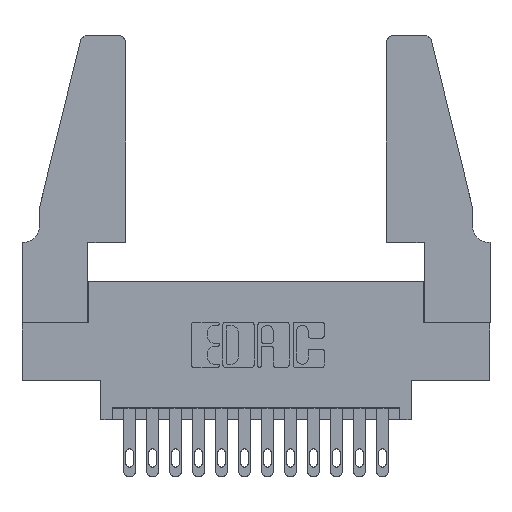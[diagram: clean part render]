
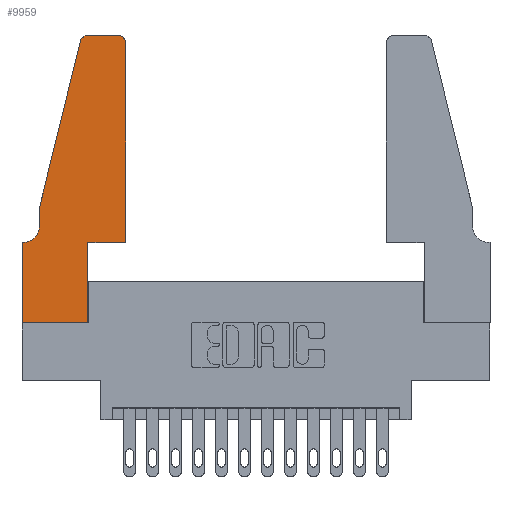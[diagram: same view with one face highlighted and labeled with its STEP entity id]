
A CAD part, top view. The second image highlights one B-rep face of the part: STEP entity #9959.
In plain terms, the highlighted planar face has unit normal (0, 0, 1).
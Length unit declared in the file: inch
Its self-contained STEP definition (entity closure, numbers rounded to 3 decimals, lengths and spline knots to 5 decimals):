
#81 = EDGE_CURVE ( 'NONE', #7477, #2497, #8953, .T. ) ;
#582 = ORIENTED_EDGE ( 'NONE', *, *, #3289, .T. ) ;
#602 = ORIENTED_EDGE ( 'NONE', *, *, #713, .T. ) ;
#713 = EDGE_CURVE ( 'NONE', #14682, #7477, #11780, .T. ) ;
#714 = PLANE ( 'NONE',  #820 ) ;
#746 = LINE ( 'NONE', #6667, #15340 ) ;
#820 = AXIS2_PLACEMENT_3D ( 'NONE', #15284, #14021, #11744 ) ;
#969 = DIRECTION ( 'NONE',  ( 1., 0., 0. ) ) ;
#1720 = CARTESIAN_POINT ( 'NONE',  ( 0.0055, 0.42, 0.37 ) ) ;
#1726 = CARTESIAN_POINT ( 'NONE',  ( 0.2865, 0.35, 0.37 ) ) ;
#1733 = EDGE_CURVE ( 'NONE', #10655, #14813, #12860, .T. ) ;
#1747 = ORIENTED_EDGE ( 'NONE', *, *, #14807, .T. ) ;
#1910 = CIRCLE ( 'NONE', #2543, 0.03 ) ;
#1950 = FACE_OUTER_BOUND ( 'NONE', #2334, .T. ) ;
#2334 = EDGE_LOOP ( 'NONE', ( #6876, #14198, #11317, #602, #5118, #5185, #582, #6405, #6562, #12380, #1747, #8671 ) ) ;
#2339 = VERTEX_POINT ( 'NONE', #14355 ) ;
#2362 = DIRECTION ( 'NONE',  ( 1., 0., 0. ) ) ;
#2379 = EDGE_CURVE ( 'NONE', #2339, #4622, #3579, .T. ) ;
#2497 = VERTEX_POINT ( 'NONE', #14504 ) ;
#2543 = AXIS2_PLACEMENT_3D ( 'NONE', #4856, #8534, #2362 ) ;
#2644 = VECTOR ( 'NONE', #969, 39.37008 ) ;
#3289 = EDGE_CURVE ( 'NONE', #13459, #10655, #746, .T. ) ;
#3384 = LINE ( 'NONE', #5779, #15113 ) ;
#3412 = DIRECTION ( 'NONE',  ( -1., 0., 0. ) ) ;
#3437 = VECTOR ( 'NONE', #10506, 39.37008 ) ;
#3526 = EDGE_CURVE ( 'NONE', #9726, #8378, #5277, .T. ) ;
#3579 = CIRCLE ( 'NONE', #4833, 0.03 ) ;
#3986 = CARTESIAN_POINT ( 'NONE',  ( 0.0755, 0.42, 0.37 ) ) ;
#4255 = LINE ( 'NONE', #6938, #6357 ) ;
#4392 = DIRECTION ( 'NONE',  ( 1., 0., 0. ) ) ;
#4622 = VERTEX_POINT ( 'NONE', #6250 ) ;
#4772 = CARTESIAN_POINT ( 'NONE',  ( 0.4505, 0.35, 0.37 ) ) ;
#4833 = AXIS2_PLACEMENT_3D ( 'NONE', #8359, #11648, #4392 ) ;
#4856 = CARTESIAN_POINT ( 'NONE',  ( 0.284, 1.22, 0.37 ) ) ;
#5118 = ORIENTED_EDGE ( 'NONE', *, *, #81, .T. ) ;
#5185 = ORIENTED_EDGE ( 'NONE', *, *, #6138, .T. ) ;
#5277 = LINE ( 'NONE', #6906, #11356 ) ;
#5686 = DIRECTION ( 'NONE',  ( 0., -1., 0. ) ) ;
#5779 = CARTESIAN_POINT ( 'NONE',  ( 0.2605, 1.25, 0.37 ) ) ;
#5795 = CARTESIAN_POINT ( 'NONE',  ( 0., 0., 0.37 ) ) ;
#5991 = LINE ( 'NONE', #15355, #14851 ) ;
#5999 = DIRECTION ( 'NONE',  ( 0., 1., 0. ) ) ;
#6138 = EDGE_CURVE ( 'NONE', #2497, #13459, #5991, .T. ) ;
#6250 = CARTESIAN_POINT ( 'NONE',  ( 0.4205, 1.25, 0.37 ) ) ;
#6342 = EDGE_CURVE ( 'NONE', #13863, #14682, #4255, .T. ) ;
#6357 = VECTOR ( 'NONE', #10728, 39.37008 ) ;
#6405 = ORIENTED_EDGE ( 'NONE', *, *, #1733, .T. ) ;
#6513 = DIRECTION ( 'NONE',  ( 0., 1., 0. ) ) ;
#6562 = ORIENTED_EDGE ( 'NONE', *, *, #8147, .T. ) ;
#6667 = CARTESIAN_POINT ( 'NONE',  ( 0., 0., 0.37 ) ) ;
#6869 = CARTESIAN_POINT ( 'NONE',  ( 0.2865, 0., 0.37 ) ) ;
#6876 = ORIENTED_EDGE ( 'NONE', *, *, #13393, .T. ) ;
#6906 = CARTESIAN_POINT ( 'NONE',  ( 0.4505, 0.35, 0.37 ) ) ;
#6938 = CARTESIAN_POINT ( 'NONE',  ( 0.0755, 0.5, 0.37 ) ) ;
#6979 = CARTESIAN_POINT ( 'NONE',  ( 0.2865, 0.35, 0.37 ) ) ;
#7275 = AXIS2_PLACEMENT_3D ( 'NONE', #1720, #10667, #3412 ) ;
#7477 = VERTEX_POINT ( 'NONE', #3986 ) ;
#7820 = LINE ( 'NONE', #1726, #13453 ) ;
#8109 = VERTEX_POINT ( 'NONE', #9934 ) ;
#8147 = EDGE_CURVE ( 'NONE', #14813, #9726, #7820, .T. ) ;
#8359 = CARTESIAN_POINT ( 'NONE',  ( 0.4205, 1.22, 0.37 ) ) ;
#8378 = VERTEX_POINT ( 'NONE', #14667 ) ;
#8495 = EDGE_CURVE ( 'NONE', #8109, #13863, #1910, .T. ) ;
#8534 = DIRECTION ( 'NONE',  ( 0., 0., 1. ) ) ;
#8671 = ORIENTED_EDGE ( 'NONE', *, *, #2379, .T. ) ;
#8953 = CIRCLE ( 'NONE', #7275, 0.07 ) ;
#9319 = CARTESIAN_POINT ( 'NONE',  ( 0., 0., 0.37 ) ) ;
#9726 = VERTEX_POINT ( 'NONE', #6979 ) ;
#9934 = CARTESIAN_POINT ( 'NONE',  ( 0.284, 1.25, 0.37 ) ) ;
#9959 = ADVANCED_FACE ( 'NONE', ( #1950 ), #714, .T. ) ;
#10326 = CARTESIAN_POINT ( 'NONE',  ( 0.0755, 0.5, 0.37 ) ) ;
#10420 = DIRECTION ( 'NONE',  ( 1., 0., 0. ) ) ;
#10506 = DIRECTION ( 'NONE',  ( 0., -1., 0. ) ) ;
#10655 = VERTEX_POINT ( 'NONE', #5795 ) ;
#10667 = DIRECTION ( 'NONE',  ( 0., 0., -1. ) ) ;
#10700 = DIRECTION ( 'NONE',  ( -1., 0., 0. ) ) ;
#10728 = DIRECTION ( 'NONE',  ( -0.239, -0.971, 0. ) ) ;
#11110 = CARTESIAN_POINT ( 'NONE',  ( 0.25487, 1.22718, 0.37 ) ) ;
#11317 = ORIENTED_EDGE ( 'NONE', *, *, #6342, .T. ) ;
#11356 = VECTOR ( 'NONE', #10420, 39.37008 ) ;
#11648 = DIRECTION ( 'NONE',  ( 0., 0., 1. ) ) ;
#11744 = DIRECTION ( 'NONE',  ( 1., 0., 0. ) ) ;
#11780 = LINE ( 'NONE', #15098, #3437 ) ;
#12178 = CARTESIAN_POINT ( 'NONE',  ( 0., 0.35, 0.37 ) ) ;
#12380 = ORIENTED_EDGE ( 'NONE', *, *, #3526, .T. ) ;
#12860 = LINE ( 'NONE', #9319, #2644 ) ;
#13393 = EDGE_CURVE ( 'NONE', #4622, #8109, #3384, .T. ) ;
#13453 = VECTOR ( 'NONE', #6513, 39.37008 ) ;
#13459 = VERTEX_POINT ( 'NONE', #12178 ) ;
#13863 = VERTEX_POINT ( 'NONE', #11110 ) ;
#14021 = DIRECTION ( 'NONE',  ( 0., 0., 1. ) ) ;
#14198 = ORIENTED_EDGE ( 'NONE', *, *, #8495, .T. ) ;
#14303 = VECTOR ( 'NONE', #5999, 39.37008 ) ;
#14355 = CARTESIAN_POINT ( 'NONE',  ( 0.4505, 1.22, 0.37 ) ) ;
#14504 = CARTESIAN_POINT ( 'NONE',  ( 0.0055, 0.35, 0.37 ) ) ;
#14667 = CARTESIAN_POINT ( 'NONE',  ( 0.4505, 0.35, 0.37 ) ) ;
#14677 = LINE ( 'NONE', #4772, #14303 ) ;
#14682 = VERTEX_POINT ( 'NONE', #10326 ) ;
#14807 = EDGE_CURVE ( 'NONE', #8378, #2339, #14677, .T. ) ;
#14813 = VERTEX_POINT ( 'NONE', #6869 ) ;
#14851 = VECTOR ( 'NONE', #15194, 39.37008 ) ;
#15098 = CARTESIAN_POINT ( 'NONE',  ( 0.0755, 0.5, 0.37 ) ) ;
#15113 = VECTOR ( 'NONE', #10700, 39.37008 ) ;
#15194 = DIRECTION ( 'NONE',  ( -1., 0., 0. ) ) ;
#15284 = CARTESIAN_POINT ( 'NONE',  ( 0., 0.35, 0.37 ) ) ;
#15340 = VECTOR ( 'NONE', #5686, 39.37008 ) ;
#15355 = CARTESIAN_POINT ( 'NONE',  ( 0.0755, 0.35, 0.37 ) ) ;
